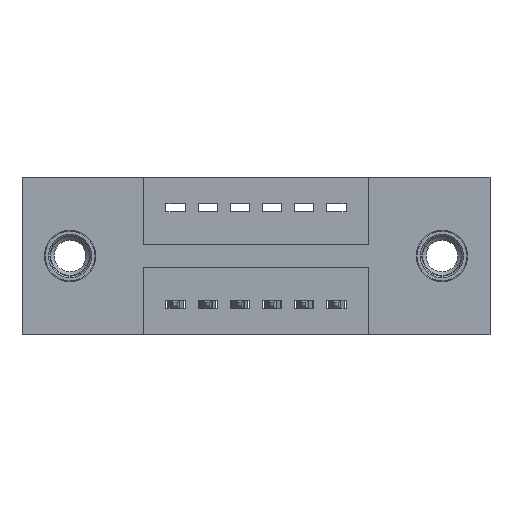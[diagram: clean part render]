
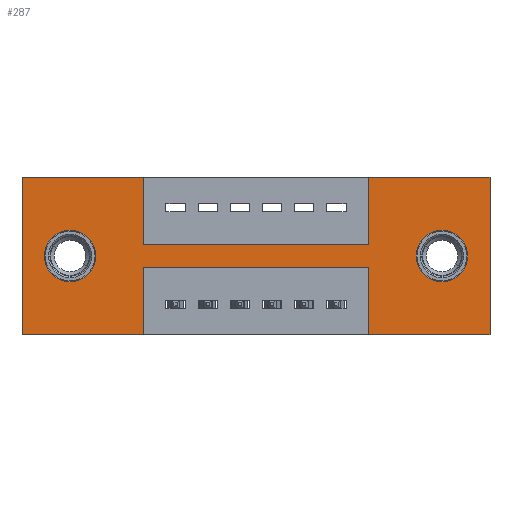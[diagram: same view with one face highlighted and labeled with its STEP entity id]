
A CAD part, front view. The second image highlights one B-rep face of the part: STEP entity #287.
In plain terms, the highlighted planar face has unit normal (0, -1, 0).
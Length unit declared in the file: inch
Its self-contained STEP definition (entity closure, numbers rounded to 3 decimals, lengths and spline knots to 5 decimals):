
#30 = EDGE_CURVE ( 'NONE', #4115, #1352, #1618, .T. ) ;
#93 = CARTESIAN_POINT ( 'NONE',  ( 0., 0., -0.49 ) ) ;
#113 = DIRECTION ( 'NONE',  ( 0., 1., 0. ) ) ;
#135 = CARTESIAN_POINT ( 'NONE',  ( 0.3775, 0., -0.21 ) ) ;
#283 = EDGE_CURVE ( 'NONE', #5102, #7330, #8640, .T. ) ;
#287 = ADVANCED_FACE ( 'NONE', ( #3019, #4498, #2549 ), #5711, .T. ) ;
#315 = CARTESIAN_POINT ( 'NONE',  ( 0., 0., 0. ) ) ;
#455 = EDGE_CURVE ( 'NONE', #9295, #6318, #6652, .T. ) ;
#461 = LINE ( 'NONE', #5642, #2674 ) ;
#641 = EDGE_CURVE ( 'NONE', #2737, #6574, #5056, .T. ) ;
#651 = VECTOR ( 'NONE', #7784, 39.37008 ) ;
#664 = VECTOR ( 'NONE', #1703, 39.37008 ) ;
#678 = CARTESIAN_POINT ( 'NONE',  ( 0.3775, 0., -0.21 ) ) ;
#774 = CARTESIAN_POINT ( 'NONE',  ( 0.3775, 0., -0.21 ) ) ;
#939 = LINE ( 'NONE', #2750, #7035 ) ;
#989 = DIRECTION ( 'NONE',  ( 0., 0., 1. ) ) ;
#1011 = CARTESIAN_POINT ( 'NONE',  ( 1.3055, 0., -0.165 ) ) ;
#1093 = CARTESIAN_POINT ( 'NONE',  ( 0., 0., -0.49 ) ) ;
#1280 = EDGE_CURVE ( 'NONE', #5992, #4115, #4146, .T. ) ;
#1352 = VERTEX_POINT ( 'NONE', #93 ) ;
#1415 = EDGE_CURVE ( 'NONE', #1352, #3265, #8731, .T. ) ;
#1551 = CARTESIAN_POINT ( 'NONE',  ( 0.1495, 0., -0.165 ) ) ;
#1618 = LINE ( 'NONE', #9545, #5297 ) ;
#1703 = DIRECTION ( 'NONE',  ( 0., 0., -1. ) ) ;
#1849 = DIRECTION ( 'NONE',  ( 0., 1., 0. ) ) ;
#1888 = DIRECTION ( 'NONE',  ( 1., 0., 0. ) ) ;
#1951 = ORIENTED_EDGE ( 'NONE', *, *, #7354, .F. ) ;
#1973 = VERTEX_POINT ( 'NONE', #4689 ) ;
#2192 = EDGE_CURVE ( 'NONE', #6574, #2737, #3636, .T. ) ;
#2207 = CARTESIAN_POINT ( 'NONE',  ( 1.455, 0., -0.49 ) ) ;
#2225 = DIRECTION ( 'NONE',  ( 0., -1., 0. ) ) ;
#2242 = ORIENTED_EDGE ( 'NONE', *, *, #4351, .F. ) ;
#2302 = CARTESIAN_POINT ( 'NONE',  ( 0., 0., 0. ) ) ;
#2447 = DIRECTION ( 'NONE',  ( 0., 0., -1. ) ) ;
#2498 = EDGE_LOOP ( 'NONE', ( #5544, #3939 ) ) ;
#2549 = FACE_OUTER_BOUND ( 'NONE', #7072, .T. ) ;
#2603 = ORIENTED_EDGE ( 'NONE', *, *, #641, .T. ) ;
#2635 = ORIENTED_EDGE ( 'NONE', *, *, #7938, .F. ) ;
#2674 = VECTOR ( 'NONE', #7850, 39.37008 ) ;
#2676 = ORIENTED_EDGE ( 'NONE', *, *, #283, .F. ) ;
#2691 = CARTESIAN_POINT ( 'NONE',  ( 1.0775, 0., 0. ) ) ;
#2735 = EDGE_CURVE ( 'NONE', #9352, #5348, #4667, .T. ) ;
#2737 = VERTEX_POINT ( 'NONE', #8781 ) ;
#2750 = CARTESIAN_POINT ( 'NONE',  ( 1.0775, 0., -0.21 ) ) ;
#2855 = AXIS2_PLACEMENT_3D ( 'NONE', #3316, #1849, #6138 ) ;
#2858 = CARTESIAN_POINT ( 'NONE',  ( 1.0775, 0., -0.21 ) ) ;
#2940 = ORIENTED_EDGE ( 'NONE', *, *, #2192, .T. ) ;
#3017 = CARTESIAN_POINT ( 'NONE',  ( 0.3775, 0., 0. ) ) ;
#3019 = FACE_BOUND ( 'NONE', #4302, .T. ) ;
#3058 = AXIS2_PLACEMENT_3D ( 'NONE', #8603, #4904, #4237 ) ;
#3077 = CARTESIAN_POINT ( 'NONE',  ( 1.3055, 0., -0.245 ) ) ;
#3104 = DIRECTION ( 'NONE',  ( -1., 0., 0. ) ) ;
#3141 = LINE ( 'NONE', #2302, #5068 ) ;
#3209 = ORIENTED_EDGE ( 'NONE', *, *, #30, .F. ) ;
#3265 = VERTEX_POINT ( 'NONE', #8945 ) ;
#3316 = CARTESIAN_POINT ( 'NONE',  ( 1.3055, 0., -0.245 ) ) ;
#3390 = EDGE_CURVE ( 'NONE', #6318, #9160, #4988, .T. ) ;
#3636 = CIRCLE ( 'NONE', #2855, 0.08 ) ;
#3642 = VERTEX_POINT ( 'NONE', #2691 ) ;
#3684 = EDGE_CURVE ( 'NONE', #5348, #9352, #4421, .T. ) ;
#3768 = DIRECTION ( 'NONE',  ( 0., 0., -1. ) ) ;
#3835 = LINE ( 'NONE', #6832, #6337 ) ;
#3909 = DIRECTION ( 'NONE',  ( 0., 1., 0. ) ) ;
#3939 = ORIENTED_EDGE ( 'NONE', *, *, #2735, .T. ) ;
#4115 = VERTEX_POINT ( 'NONE', #6036 ) ;
#4146 = LINE ( 'NONE', #6788, #664 ) ;
#4162 = EDGE_CURVE ( 'NONE', #1973, #5102, #3835, .T. ) ;
#4237 = DIRECTION ( 'NONE',  ( 0., 0., 1. ) ) ;
#4247 = CARTESIAN_POINT ( 'NONE',  ( 0.3775, 0., -0.28 ) ) ;
#4302 = EDGE_LOOP ( 'NONE', ( #2940, #2603 ) ) ;
#4351 = EDGE_CURVE ( 'NONE', #9160, #3642, #939, .T. ) ;
#4421 = CIRCLE ( 'NONE', #3058, 0.08 ) ;
#4498 = FACE_BOUND ( 'NONE', #2498, .T. ) ;
#4650 = ORIENTED_EDGE ( 'NONE', *, *, #1280, .F. ) ;
#4667 = CIRCLE ( 'NONE', #6282, 0.08 ) ;
#4689 = CARTESIAN_POINT ( 'NONE',  ( 1.455, 0., 0. ) ) ;
#4707 = VECTOR ( 'NONE', #6164, 39.37008 ) ;
#4851 = EDGE_CURVE ( 'NONE', #3265, #9295, #4907, .T. ) ;
#4904 = DIRECTION ( 'NONE',  ( 0., 1., 0. ) ) ;
#4907 = LINE ( 'NONE', #7550, #7320 ) ;
#4988 = LINE ( 'NONE', #135, #8447 ) ;
#4997 = ORIENTED_EDGE ( 'NONE', *, *, #1415, .F. ) ;
#5056 = CIRCLE ( 'NONE', #5590, 0.08 ) ;
#5068 = VECTOR ( 'NONE', #5167, 39.37008 ) ;
#5102 = VERTEX_POINT ( 'NONE', #2207 ) ;
#5167 = DIRECTION ( 'NONE',  ( 1., 0., 0. ) ) ;
#5297 = VECTOR ( 'NONE', #3104, 39.37008 ) ;
#5348 = VERTEX_POINT ( 'NONE', #1551 ) ;
#5499 = CARTESIAN_POINT ( 'NONE',  ( 1.0775, 0., -0.49 ) ) ;
#5544 = ORIENTED_EDGE ( 'NONE', *, *, #3684, .T. ) ;
#5590 = AXIS2_PLACEMENT_3D ( 'NONE', #3077, #113, #3768 ) ;
#5642 = CARTESIAN_POINT ( 'NONE',  ( 1.0775, 0., -0.28 ) ) ;
#5711 = PLANE ( 'NONE',  #9194 ) ;
#5965 = VECTOR ( 'NONE', #8177, 39.37008 ) ;
#5992 = VERTEX_POINT ( 'NONE', #8269 ) ;
#6036 = CARTESIAN_POINT ( 'NONE',  ( 0.3775, 0., -0.49 ) ) ;
#6040 = CARTESIAN_POINT ( 'NONE',  ( 0.1495, 0., -0.325 ) ) ;
#6048 = ORIENTED_EDGE ( 'NONE', *, *, #4851, .F. ) ;
#6130 = DIRECTION ( 'NONE',  ( -1., 0., 0. ) ) ;
#6138 = DIRECTION ( 'NONE',  ( 0., 0., -1. ) ) ;
#6164 = DIRECTION ( 'NONE',  ( 0., 0., 1. ) ) ;
#6282 = AXIS2_PLACEMENT_3D ( 'NONE', #6699, #3909, #989 ) ;
#6318 = VERTEX_POINT ( 'NONE', #678 ) ;
#6337 = VECTOR ( 'NONE', #2447, 39.37008 ) ;
#6423 = VECTOR ( 'NONE', #6130, 39.37008 ) ;
#6479 = VERTEX_POINT ( 'NONE', #7450 ) ;
#6574 = VERTEX_POINT ( 'NONE', #1011 ) ;
#6652 = LINE ( 'NONE', #774, #5965 ) ;
#6699 = CARTESIAN_POINT ( 'NONE',  ( 0.1495, 0., -0.245 ) ) ;
#6757 = LINE ( 'NONE', #4247, #651 ) ;
#6788 = CARTESIAN_POINT ( 'NONE',  ( 0.3775, 0., -0.28 ) ) ;
#6832 = CARTESIAN_POINT ( 'NONE',  ( 1.455, 0., 0. ) ) ;
#7035 = VECTOR ( 'NONE', #7821, 39.37008 ) ;
#7072 = EDGE_LOOP ( 'NONE', ( #2242, #7091, #7909, #6048, #4997, #3209, #4650, #9166, #1951, #2676, #7342, #2635 ) ) ;
#7091 = ORIENTED_EDGE ( 'NONE', *, *, #3390, .F. ) ;
#7202 = CARTESIAN_POINT ( 'NONE',  ( 0., 0., -0.49 ) ) ;
#7320 = VECTOR ( 'NONE', #1888, 39.37008 ) ;
#7330 = VERTEX_POINT ( 'NONE', #5499 ) ;
#7342 = ORIENTED_EDGE ( 'NONE', *, *, #4162, .F. ) ;
#7354 = EDGE_CURVE ( 'NONE', #7330, #6479, #461, .T. ) ;
#7450 = CARTESIAN_POINT ( 'NONE',  ( 1.0775, 0., -0.28 ) ) ;
#7550 = CARTESIAN_POINT ( 'NONE',  ( 0., 0., 0. ) ) ;
#7784 = DIRECTION ( 'NONE',  ( -1., 0., 0. ) ) ;
#7821 = DIRECTION ( 'NONE',  ( 0., 0., 1. ) ) ;
#7850 = DIRECTION ( 'NONE',  ( 0., 0., 1. ) ) ;
#7909 = ORIENTED_EDGE ( 'NONE', *, *, #455, .F. ) ;
#7938 = EDGE_CURVE ( 'NONE', #3642, #1973, #3141, .T. ) ;
#8167 = DIRECTION ( 'NONE',  ( 1., 0., 0. ) ) ;
#8177 = DIRECTION ( 'NONE',  ( 0., 0., -1. ) ) ;
#8269 = CARTESIAN_POINT ( 'NONE',  ( 0.3775, 0., -0.28 ) ) ;
#8432 = EDGE_CURVE ( 'NONE', #6479, #5992, #6757, .T. ) ;
#8447 = VECTOR ( 'NONE', #8167, 39.37008 ) ;
#8603 = CARTESIAN_POINT ( 'NONE',  ( 0.1495, 0., -0.245 ) ) ;
#8640 = LINE ( 'NONE', #1093, #6423 ) ;
#8731 = LINE ( 'NONE', #315, #4707 ) ;
#8781 = CARTESIAN_POINT ( 'NONE',  ( 1.3055, 0., -0.325 ) ) ;
#8848 = DIRECTION ( 'NONE',  ( 0., 0., -1. ) ) ;
#8945 = CARTESIAN_POINT ( 'NONE',  ( 0., 0., 0. ) ) ;
#9160 = VERTEX_POINT ( 'NONE', #2858 ) ;
#9166 = ORIENTED_EDGE ( 'NONE', *, *, #8432, .F. ) ;
#9194 = AXIS2_PLACEMENT_3D ( 'NONE', #7202, #2225, #8848 ) ;
#9295 = VERTEX_POINT ( 'NONE', #3017 ) ;
#9352 = VERTEX_POINT ( 'NONE', #6040 ) ;
#9545 = CARTESIAN_POINT ( 'NONE',  ( 0., 0., -0.49 ) ) ;
